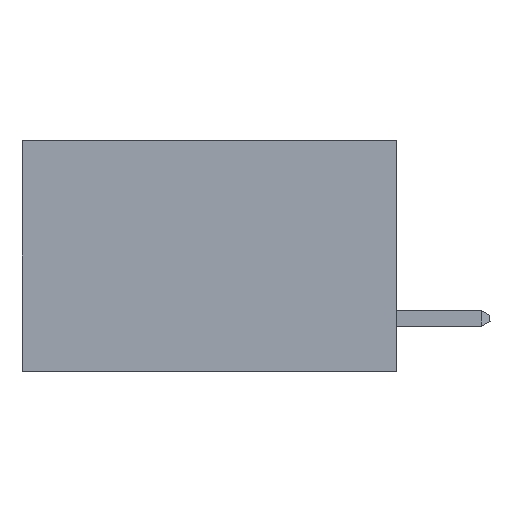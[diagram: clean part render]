
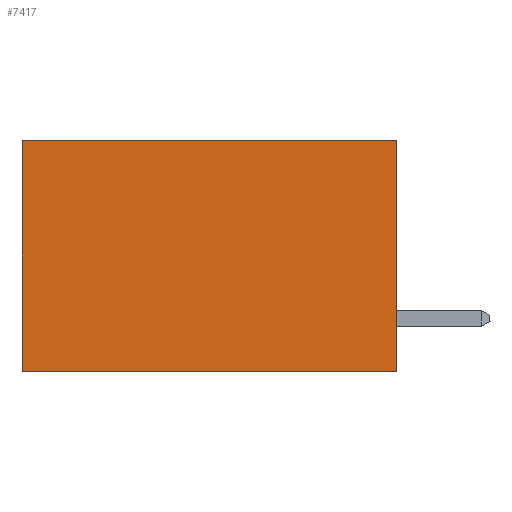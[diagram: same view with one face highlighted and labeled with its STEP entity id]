
A CAD part, left-side view. The second image highlights one B-rep face of the part: STEP entity #7417.
In plain terms, the highlighted planar face has unit normal (-1, 0, 0).
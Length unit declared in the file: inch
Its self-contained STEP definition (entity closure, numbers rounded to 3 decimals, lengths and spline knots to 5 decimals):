
#161 = ORIENTED_EDGE ( 'NONE', *, *, #14232, .F. ) ;
#320 = VERTEX_POINT ( 'NONE', #4968 ) ;
#418 = VERTEX_POINT ( 'NONE', #14356 ) ;
#2981 = VECTOR ( 'NONE', #17567, 39.37008 ) ;
#3790 = VECTOR ( 'NONE', #9037, 39.37008 ) ;
#3817 = VECTOR ( 'NONE', #7909, 39.37008 ) ;
#4968 = CARTESIAN_POINT ( 'NONE',  ( 0.298, 0.6, -0.37 ) ) ;
#5016 = ORIENTED_EDGE ( 'NONE', *, *, #21493, .T. ) ;
#6145 = CARTESIAN_POINT ( 'NONE',  ( 0.298, 0., 0. ) ) ;
#7001 = VECTOR ( 'NONE', #9728, 39.37008 ) ;
#7185 = VERTEX_POINT ( 'NONE', #18583 ) ;
#7417 = ADVANCED_FACE ( 'NONE', ( #20084 ), #15502, .F. ) ;
#7909 = DIRECTION ( 'NONE',  ( 0., 0., -1. ) ) ;
#7984 = CARTESIAN_POINT ( 'NONE',  ( 0.298, 0., 0. ) ) ;
#8442 = LINE ( 'NONE', #6145, #3817 ) ;
#8963 = CARTESIAN_POINT ( 'NONE',  ( 0.298, 0., -0.37 ) ) ;
#9037 = DIRECTION ( 'NONE',  ( 0., 1., 0. ) ) ;
#9044 = VERTEX_POINT ( 'NONE', #10616 ) ;
#9728 = DIRECTION ( 'NONE',  ( 0., 1., 0. ) ) ;
#9890 = EDGE_CURVE ( 'NONE', #7185, #320, #17523, .T. ) ;
#10616 = CARTESIAN_POINT ( 'NONE',  ( 0.298, 0., 0. ) ) ;
#10660 = ORIENTED_EDGE ( 'NONE', *, *, #20221, .T. ) ;
#11809 = DIRECTION ( 'NONE',  ( 1., 0., 0. ) ) ;
#13404 = EDGE_LOOP ( 'NONE', ( #10660, #17970, #161, #5016 ) ) ;
#14232 = EDGE_CURVE ( 'NONE', #9044, #7185, #8442, .T. ) ;
#14356 = CARTESIAN_POINT ( 'NONE',  ( 0.298, 0.6, 0. ) ) ;
#15502 = PLANE ( 'NONE',  #21579 ) ;
#15850 = CARTESIAN_POINT ( 'NONE',  ( 0.298, 0.6, 0. ) ) ;
#16462 = CARTESIAN_POINT ( 'NONE',  ( 0.298, 0., 0. ) ) ;
#16499 = DIRECTION ( 'NONE',  ( 0., 0., -1. ) ) ;
#16679 = LINE ( 'NONE', #7984, #7001 ) ;
#16744 = LINE ( 'NONE', #15850, #2981 ) ;
#17523 = LINE ( 'NONE', #8963, #3790 ) ;
#17567 = DIRECTION ( 'NONE',  ( 0., 0., -1. ) ) ;
#17970 = ORIENTED_EDGE ( 'NONE', *, *, #9890, .F. ) ;
#18583 = CARTESIAN_POINT ( 'NONE',  ( 0.298, 0., -0.37 ) ) ;
#20084 = FACE_OUTER_BOUND ( 'NONE', #13404, .T. ) ;
#20221 = EDGE_CURVE ( 'NONE', #418, #320, #16744, .T. ) ;
#21493 = EDGE_CURVE ( 'NONE', #9044, #418, #16679, .T. ) ;
#21579 = AXIS2_PLACEMENT_3D ( 'NONE', #16462, #11809, #16499 ) ;
